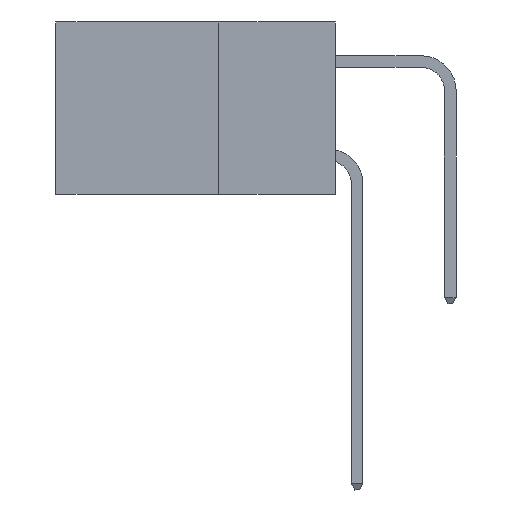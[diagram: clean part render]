
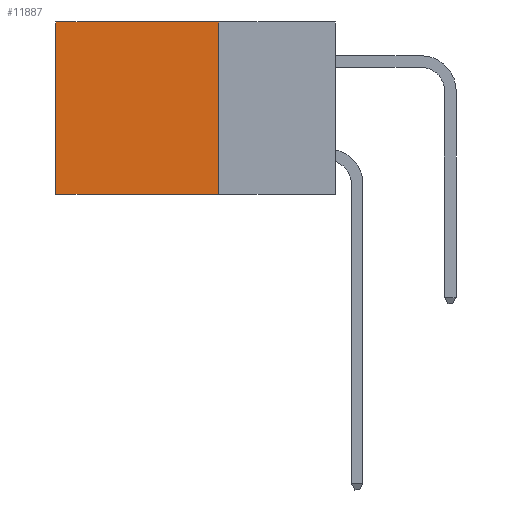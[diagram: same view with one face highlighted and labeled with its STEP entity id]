
A CAD part, left-side view. The second image highlights one B-rep face of the part: STEP entity #11887.
In plain terms, the highlighted planar face has unit normal (-1, 0, 0).
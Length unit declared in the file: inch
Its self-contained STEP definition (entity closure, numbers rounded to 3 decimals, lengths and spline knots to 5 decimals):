
#185 = ORIENTED_EDGE ( 'NONE', *, *, #1916, .F. ) ;
#501 = CARTESIAN_POINT ( 'NONE',  ( 0.2875, 0.25, 0. ) ) ;
#524 = CARTESIAN_POINT ( 'NONE',  ( 0.2875, 0.25, -0.37 ) ) ;
#641 = DIRECTION ( 'NONE',  ( 0., 0., -1. ) ) ;
#823 = DIRECTION ( 'NONE',  ( 0., 0., -1. ) ) ;
#864 = EDGE_CURVE ( 'NONE', #15009, #11155, #8455, .T. ) ;
#1074 = ORIENTED_EDGE ( 'NONE', *, *, #864, .F. ) ;
#1119 = LINE ( 'NONE', #501, #13781 ) ;
#1210 = EDGE_LOOP ( 'NONE', ( #16857, #1074, #185, #14539 ) ) ;
#1557 = CARTESIAN_POINT ( 'NONE',  ( 0.2875, 0.25, 0. ) ) ;
#1916 = EDGE_CURVE ( 'NONE', #11172, #15009, #1119, .T. ) ;
#2386 = CARTESIAN_POINT ( 'NONE',  ( 0.2875, 0.6, 0. ) ) ;
#4516 = CARTESIAN_POINT ( 'NONE',  ( 0.2875, 0.25, -0.37 ) ) ;
#5347 = LINE ( 'NONE', #2386, #12182 ) ;
#5995 = EDGE_CURVE ( 'NONE', #11172, #15398, #10777, .T. ) ;
#6009 = VECTOR ( 'NONE', #10104, 39.37008 ) ;
#6032 = FACE_OUTER_BOUND ( 'NONE', #1210, .T. ) ;
#6432 = CARTESIAN_POINT ( 'NONE',  ( 0.2875, 0.6, -0.37 ) ) ;
#8087 = VECTOR ( 'NONE', #12432, 39.37008 ) ;
#8391 = CARTESIAN_POINT ( 'NONE',  ( 0.2875, 0.25, 0. ) ) ;
#8455 = LINE ( 'NONE', #524, #6009 ) ;
#9467 = AXIS2_PLACEMENT_3D ( 'NONE', #8391, #13088, #19197 ) ;
#10104 = DIRECTION ( 'NONE',  ( 0., 1., 0. ) ) ;
#10211 = CARTESIAN_POINT ( 'NONE',  ( 0.2875, 0.6, 0. ) ) ;
#10777 = LINE ( 'NONE', #1557, #8087 ) ;
#11079 = CARTESIAN_POINT ( 'NONE',  ( 0.2875, 0.25, 0. ) ) ;
#11155 = VERTEX_POINT ( 'NONE', #6432 ) ;
#11172 = VERTEX_POINT ( 'NONE', #11079 ) ;
#11887 = ADVANCED_FACE ( 'NONE', ( #6032 ), #19336, .F. ) ;
#12182 = VECTOR ( 'NONE', #823, 39.37008 ) ;
#12432 = DIRECTION ( 'NONE',  ( 0., 1., 0. ) ) ;
#13088 = DIRECTION ( 'NONE',  ( 1., 0., 0. ) ) ;
#13781 = VECTOR ( 'NONE', #641, 39.37008 ) ;
#14539 = ORIENTED_EDGE ( 'NONE', *, *, #5995, .T. ) ;
#15009 = VERTEX_POINT ( 'NONE', #4516 ) ;
#15398 = VERTEX_POINT ( 'NONE', #10211 ) ;
#16857 = ORIENTED_EDGE ( 'NONE', *, *, #17074, .T. ) ;
#17074 = EDGE_CURVE ( 'NONE', #15398, #11155, #5347, .T. ) ;
#19197 = DIRECTION ( 'NONE',  ( 0., 0., -1. ) ) ;
#19336 = PLANE ( 'NONE',  #9467 ) ;
